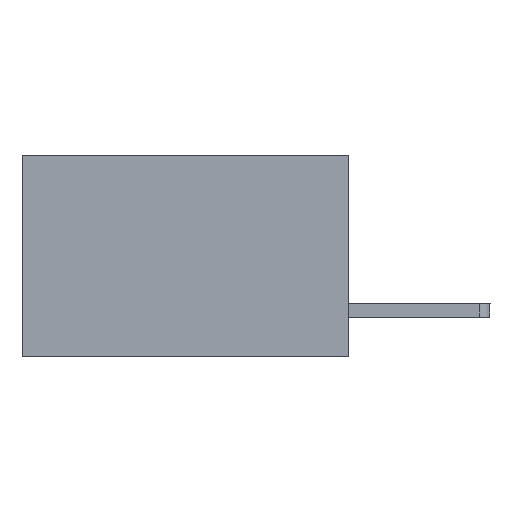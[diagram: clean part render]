
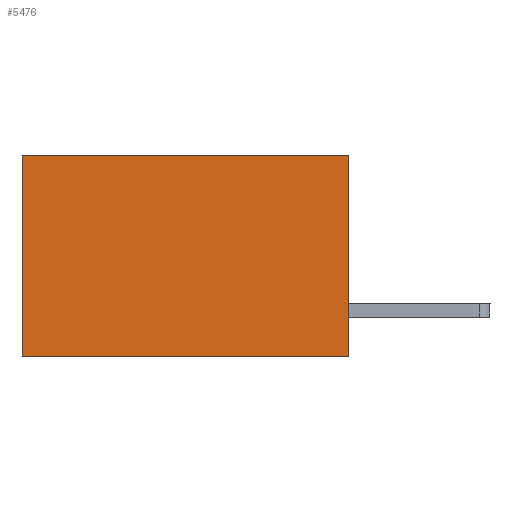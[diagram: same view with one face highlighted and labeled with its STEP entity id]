
A CAD part, left-side view. The second image highlights one B-rep face of the part: STEP entity #5476.
In plain terms, the highlighted planar face has unit normal (-1, 0, 0).
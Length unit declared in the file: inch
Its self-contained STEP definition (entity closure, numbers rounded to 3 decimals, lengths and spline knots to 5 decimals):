
#326 = CARTESIAN_POINT ( 'NONE',  ( 0.298, 0.6, 0. ) ) ;
#370 = DIRECTION ( 'NONE',  ( 0., 0., -1. ) ) ;
#402 = ORIENTED_EDGE ( 'NONE', *, *, #7247, .F. ) ;
#621 = LINE ( 'NONE', #9423, #5646 ) ;
#707 = ORIENTED_EDGE ( 'NONE', *, *, #8499, .T. ) ;
#897 = ORIENTED_EDGE ( 'NONE', *, *, #8693, .F. ) ;
#1247 = CARTESIAN_POINT ( 'NONE',  ( 0.298, 0., 0. ) ) ;
#1575 = VERTEX_POINT ( 'NONE', #9605 ) ;
#1849 = CARTESIAN_POINT ( 'NONE',  ( 0.298, 0., 0. ) ) ;
#2071 = CARTESIAN_POINT ( 'NONE',  ( 0.298, 0.6, -0.37 ) ) ;
#4276 = VECTOR ( 'NONE', #8156, 39.37008 ) ;
#4753 = VECTOR ( 'NONE', #5956, 39.37008 ) ;
#4830 = ORIENTED_EDGE ( 'NONE', *, *, #10071, .T. ) ;
#5149 = LINE ( 'NONE', #6426, #4276 ) ;
#5296 = CARTESIAN_POINT ( 'NONE',  ( 0.298, 0., 0. ) ) ;
#5476 = ADVANCED_FACE ( 'NONE', ( #7736 ), #9353, .F. ) ;
#5531 = LINE ( 'NONE', #326, #4753 ) ;
#5646 = VECTOR ( 'NONE', #10236, 39.37008 ) ;
#5956 = DIRECTION ( 'NONE',  ( 0., 0., -1. ) ) ;
#6108 = DIRECTION ( 'NONE',  ( 1., 0., 0. ) ) ;
#6256 = AXIS2_PLACEMENT_3D ( 'NONE', #5296, #6108, #370 ) ;
#6259 = VECTOR ( 'NONE', #9139, 39.37008 ) ;
#6426 = CARTESIAN_POINT ( 'NONE',  ( 0.298, 0., -0.37 ) ) ;
#7010 = VERTEX_POINT ( 'NONE', #8594 ) ;
#7247 = EDGE_CURVE ( 'NONE', #7010, #9430, #5149, .T. ) ;
#7586 = EDGE_LOOP ( 'NONE', ( #707, #402, #897, #4830 ) ) ;
#7736 = FACE_OUTER_BOUND ( 'NONE', #7586, .T. ) ;
#8156 = DIRECTION ( 'NONE',  ( 0., 1., 0. ) ) ;
#8423 = LINE ( 'NONE', #1849, #6259 ) ;
#8499 = EDGE_CURVE ( 'NONE', #1575, #9430, #5531, .T. ) ;
#8594 = CARTESIAN_POINT ( 'NONE',  ( 0.298, 0., -0.37 ) ) ;
#8693 = EDGE_CURVE ( 'NONE', #8703, #7010, #621, .T. ) ;
#8703 = VERTEX_POINT ( 'NONE', #1247 ) ;
#9139 = DIRECTION ( 'NONE',  ( 0., 1., 0. ) ) ;
#9353 = PLANE ( 'NONE',  #6256 ) ;
#9423 = CARTESIAN_POINT ( 'NONE',  ( 0.298, 0., 0. ) ) ;
#9430 = VERTEX_POINT ( 'NONE', #2071 ) ;
#9605 = CARTESIAN_POINT ( 'NONE',  ( 0.298, 0.6, 0. ) ) ;
#10071 = EDGE_CURVE ( 'NONE', #8703, #1575, #8423, .T. ) ;
#10236 = DIRECTION ( 'NONE',  ( 0., 0., -1. ) ) ;
